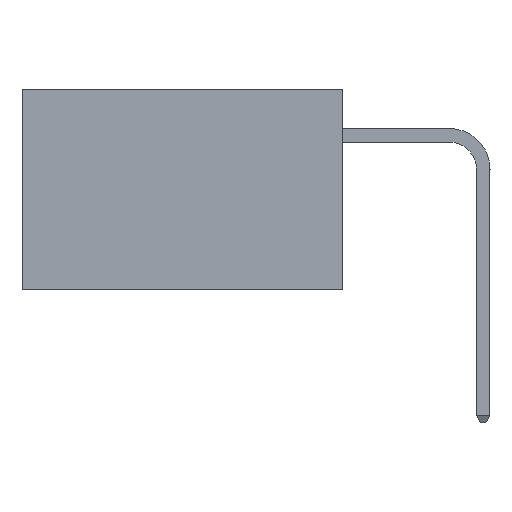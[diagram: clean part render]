
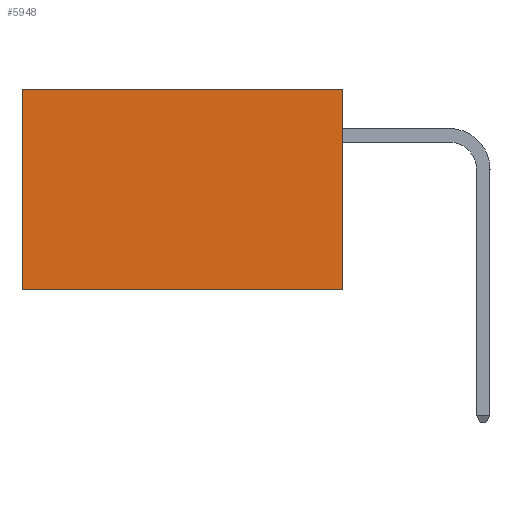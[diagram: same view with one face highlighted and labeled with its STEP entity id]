
A CAD part, left-side view. The second image highlights one B-rep face of the part: STEP entity #5948.
In plain terms, the highlighted planar face has unit normal (-1, 0, 0).
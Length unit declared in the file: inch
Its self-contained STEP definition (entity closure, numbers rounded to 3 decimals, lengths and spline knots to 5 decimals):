
#114 = DIRECTION ( 'NONE',  ( 0., 0., -1. ) ) ;
#384 = VERTEX_POINT ( 'NONE', #7642 ) ;
#992 = EDGE_CURVE ( 'NONE', #384, #2805, #8339, .T. ) ;
#1007 = CARTESIAN_POINT ( 'NONE',  ( 0.277, 0., -0.37 ) ) ;
#1167 = DIRECTION ( 'NONE',  ( 0., 1., 0. ) ) ;
#1188 = EDGE_CURVE ( 'NONE', #10046, #4865, #2509, .T. ) ;
#1406 = EDGE_CURVE ( 'NONE', #384, #10046, #8602, .T. ) ;
#1877 = DIRECTION ( 'NONE',  ( 0., 1., 0. ) ) ;
#2076 = CARTESIAN_POINT ( 'NONE',  ( 0.277, 0., -0.37 ) ) ;
#2475 = CARTESIAN_POINT ( 'NONE',  ( 0.277, 0., 0. ) ) ;
#2509 = LINE ( 'NONE', #2076, #4244 ) ;
#2805 = VERTEX_POINT ( 'NONE', #6628 ) ;
#4172 = DIRECTION ( 'NONE',  ( 1., 0., 0. ) ) ;
#4244 = VECTOR ( 'NONE', #1877, 39.37008 ) ;
#4865 = VERTEX_POINT ( 'NONE', #6314 ) ;
#5150 = CARTESIAN_POINT ( 'NONE',  ( 0.277, 0., -0.37 ) ) ;
#5901 = LINE ( 'NONE', #9835, #6467 ) ;
#5946 = VECTOR ( 'NONE', #1167, 39.37008 ) ;
#5948 = ADVANCED_FACE ( 'NONE', ( #8342 ), #7788, .F. ) ;
#6129 = EDGE_LOOP ( 'NONE', ( #7903, #7585, #7633, #7851 ) ) ;
#6314 = CARTESIAN_POINT ( 'NONE',  ( 0.277, 0.59, -0.37 ) ) ;
#6467 = VECTOR ( 'NONE', #114, 39.37008 ) ;
#6628 = CARTESIAN_POINT ( 'NONE',  ( 0.277, 0.59, 0. ) ) ;
#6862 = AXIS2_PLACEMENT_3D ( 'NONE', #9509, #4172, #10371 ) ;
#7585 = ORIENTED_EDGE ( 'NONE', *, *, #1188, .F. ) ;
#7633 = ORIENTED_EDGE ( 'NONE', *, *, #1406, .F. ) ;
#7642 = CARTESIAN_POINT ( 'NONE',  ( 0.277, 0., 0. ) ) ;
#7788 = PLANE ( 'NONE',  #6862 ) ;
#7851 = ORIENTED_EDGE ( 'NONE', *, *, #992, .T. ) ;
#7903 = ORIENTED_EDGE ( 'NONE', *, *, #8727, .T. ) ;
#8339 = LINE ( 'NONE', #2475, #5946 ) ;
#8342 = FACE_OUTER_BOUND ( 'NONE', #6129, .T. ) ;
#8602 = LINE ( 'NONE', #1007, #11074 ) ;
#8727 = EDGE_CURVE ( 'NONE', #2805, #4865, #5901, .T. ) ;
#9509 = CARTESIAN_POINT ( 'NONE',  ( 0.277, 0., -0.37 ) ) ;
#9632 = DIRECTION ( 'NONE',  ( 0., 0., -1. ) ) ;
#9835 = CARTESIAN_POINT ( 'NONE',  ( 0.277, 0.59, -0.37 ) ) ;
#10046 = VERTEX_POINT ( 'NONE', #5150 ) ;
#10371 = DIRECTION ( 'NONE',  ( 0., 0., -1. ) ) ;
#11074 = VECTOR ( 'NONE', #9632, 39.37008 ) ;
